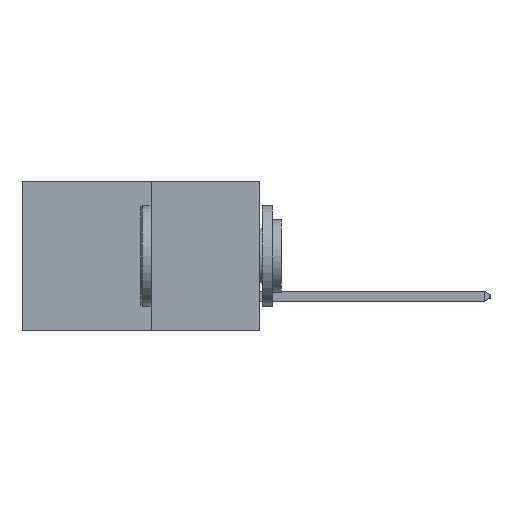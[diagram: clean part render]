
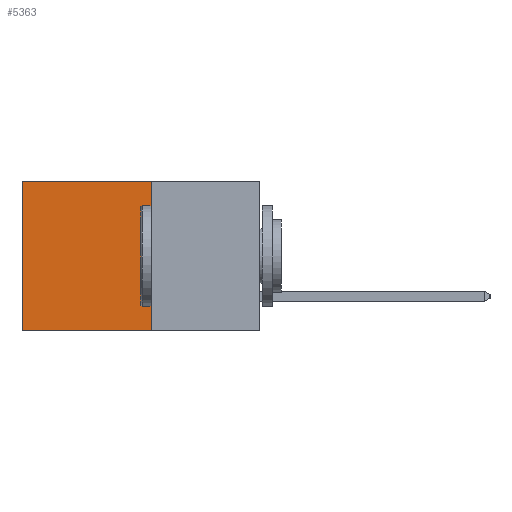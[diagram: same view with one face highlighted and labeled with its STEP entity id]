
A CAD part, left-side view. The second image highlights one B-rep face of the part: STEP entity #5363.
In plain terms, the highlighted planar face has unit normal (-1, 0, 0).
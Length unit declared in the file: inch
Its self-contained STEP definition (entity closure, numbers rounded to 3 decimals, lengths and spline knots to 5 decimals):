
#1319 = VERTEX_POINT ( 'NONE', #18504 ) ;
#2818 = VECTOR ( 'NONE', #13343, 39.37008 ) ;
#2950 = VERTEX_POINT ( 'NONE', #11513 ) ;
#3152 = LINE ( 'NONE', #6767, #14467 ) ;
#3907 = EDGE_CURVE ( 'NONE', #1319, #2950, #10003, .T. ) ;
#5363 = ADVANCED_FACE ( 'NONE', ( #23363 ), #13127, .F. ) ;
#6767 = CARTESIAN_POINT ( 'NONE',  ( 0.277, 0.59, -0.37 ) ) ;
#6816 = EDGE_CURVE ( 'NONE', #13381, #1319, #22065, .T. ) ;
#7719 = CARTESIAN_POINT ( 'NONE',  ( 0.277, 0.27, -0.37 ) ) ;
#8345 = LINE ( 'NONE', #24982, #2818 ) ;
#9733 = DIRECTION ( 'NONE',  ( 0., 0., -1. ) ) ;
#10003 = LINE ( 'NONE', #12820, #20968 ) ;
#10187 = EDGE_CURVE ( 'NONE', #14260, #2950, #3152, .T. ) ;
#10383 = EDGE_CURVE ( 'NONE', #13381, #14260, #8345, .T. ) ;
#10540 = ORIENTED_EDGE ( 'NONE', *, *, #6816, .F. ) ;
#11513 = CARTESIAN_POINT ( 'NONE',  ( 0.277, 0.59, -0.37 ) ) ;
#12498 = AXIS2_PLACEMENT_3D ( 'NONE', #13373, #13039, #13010 ) ;
#12820 = CARTESIAN_POINT ( 'NONE',  ( 0.277, 0.27, -0.37 ) ) ;
#13010 = DIRECTION ( 'NONE',  ( 0., 0., -1. ) ) ;
#13039 = DIRECTION ( 'NONE',  ( 1., 0., 0. ) ) ;
#13127 = PLANE ( 'NONE',  #12498 ) ;
#13129 = DIRECTION ( 'NONE',  ( 0., 1., 0. ) ) ;
#13343 = DIRECTION ( 'NONE',  ( 0., 1., 0. ) ) ;
#13373 = CARTESIAN_POINT ( 'NONE',  ( 0.277, 0.27, -0.37 ) ) ;
#13381 = VERTEX_POINT ( 'NONE', #23500 ) ;
#14260 = VERTEX_POINT ( 'NONE', #16841 ) ;
#14467 = VECTOR ( 'NONE', #22468, 39.37008 ) ;
#16841 = CARTESIAN_POINT ( 'NONE',  ( 0.277, 0.59, 0. ) ) ;
#18504 = CARTESIAN_POINT ( 'NONE',  ( 0.277, 0.27, -0.37 ) ) ;
#18998 = ORIENTED_EDGE ( 'NONE', *, *, #10383, .T. ) ;
#20968 = VECTOR ( 'NONE', #13129, 39.37008 ) ;
#21461 = VECTOR ( 'NONE', #9733, 39.37008 ) ;
#22065 = LINE ( 'NONE', #7719, #21461 ) ;
#22468 = DIRECTION ( 'NONE',  ( 0., 0., -1. ) ) ;
#23363 = FACE_OUTER_BOUND ( 'NONE', #24044, .T. ) ;
#23401 = ORIENTED_EDGE ( 'NONE', *, *, #10187, .T. ) ;
#23500 = CARTESIAN_POINT ( 'NONE',  ( 0.277, 0.27, 0. ) ) ;
#24044 = EDGE_LOOP ( 'NONE', ( #23401, #25408, #10540, #18998 ) ) ;
#24982 = CARTESIAN_POINT ( 'NONE',  ( 0.277, 0.27, 0. ) ) ;
#25408 = ORIENTED_EDGE ( 'NONE', *, *, #3907, .F. ) ;
